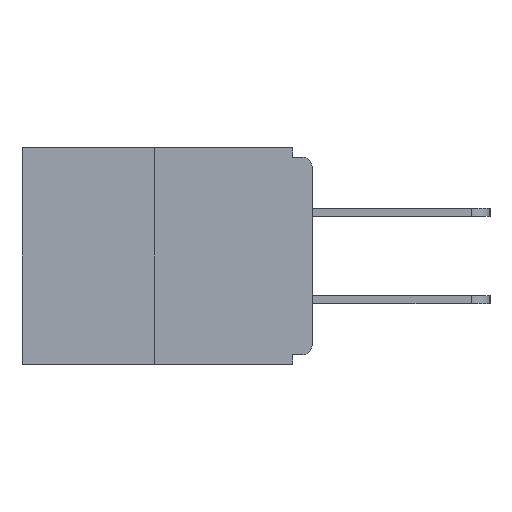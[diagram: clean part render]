
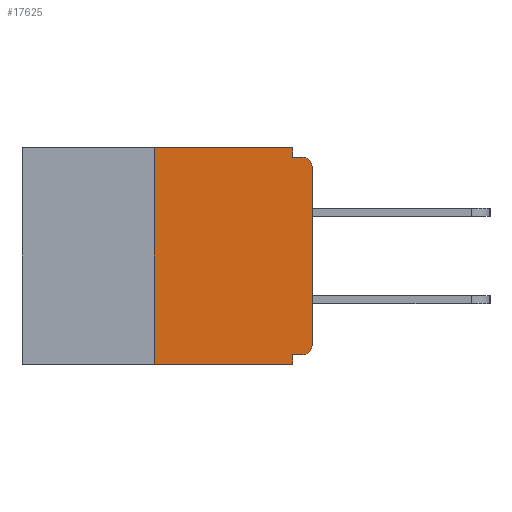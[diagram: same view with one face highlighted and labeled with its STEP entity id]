
A CAD part, left-side view. The second image highlights one B-rep face of the part: STEP entity #17625.
In plain terms, the highlighted planar face has unit normal (-1, 0, 0).
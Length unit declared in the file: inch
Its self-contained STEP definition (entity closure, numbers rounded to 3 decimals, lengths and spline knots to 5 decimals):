
#18 = EDGE_CURVE ( 'NONE', #6038, #10731, #11660, .T. ) ;
#151 = ORIENTED_EDGE ( 'NONE', *, *, #4765, .T. ) ;
#837 = EDGE_CURVE ( 'NONE', #8787, #17537, #17815, .T. ) ;
#917 = CIRCLE ( 'NONE', #1134, 0.015 ) ;
#981 = CARTESIAN_POINT ( 'NONE',  ( 0., 0.031, -0.015 ) ) ;
#1134 = AXIS2_PLACEMENT_3D ( 'NONE', #4329, #6151, #19952 ) ;
#1770 = DIRECTION ( 'NONE',  ( 0., -1., 0. ) ) ;
#2172 = CARTESIAN_POINT ( 'NONE',  ( 0., 0.46, -0.343 ) ) ;
#3503 = ORIENTED_EDGE ( 'NONE', *, *, #23563, .F. ) ;
#3613 = CARTESIAN_POINT ( 'NONE',  ( 0., 0.25, -0.343 ) ) ;
#3852 = CARTESIAN_POINT ( 'NONE',  ( 0., 0.46, 0. ) ) ;
#4032 = DIRECTION ( 'NONE',  ( 0., 0., 1. ) ) ;
#4329 = CARTESIAN_POINT ( 'NONE',  ( 0., 0.015, -0.313 ) ) ;
#4765 = EDGE_CURVE ( 'NONE', #13293, #6038, #917, .T. ) ;
#5050 = CARTESIAN_POINT ( 'NONE',  ( 0., 0.031, 0. ) ) ;
#5633 = DIRECTION ( 'NONE',  ( -1., 0., 0. ) ) ;
#5678 = CARTESIAN_POINT ( 'NONE',  ( 0., 0.015, -0.328 ) ) ;
#5703 = LINE ( 'NONE', #20568, #8484 ) ;
#5723 = EDGE_CURVE ( 'NONE', #21055, #6107, #17226, .T. ) ;
#5806 = EDGE_CURVE ( 'NONE', #13293, #19274, #21233, .T. ) ;
#6010 = CARTESIAN_POINT ( 'NONE',  ( 0., 0.46, 0. ) ) ;
#6038 = VERTEX_POINT ( 'NONE', #20214 ) ;
#6107 = VERTEX_POINT ( 'NONE', #981 ) ;
#6151 = DIRECTION ( 'NONE',  ( -1., 0., 0. ) ) ;
#6972 = DIRECTION ( 'NONE',  ( 0., 0., 1. ) ) ;
#7076 = ORIENTED_EDGE ( 'NONE', *, *, #9445, .F. ) ;
#7399 = CARTESIAN_POINT ( 'NONE',  ( 0., 0.25, 0. ) ) ;
#7522 = CARTESIAN_POINT ( 'NONE',  ( 0., 0., -0.015 ) ) ;
#7923 = VECTOR ( 'NONE', #6972, 39.37008 ) ;
#7946 = DIRECTION ( 'NONE',  ( 0., -1., 0. ) ) ;
#8337 = CARTESIAN_POINT ( 'NONE',  ( 0., 0.031, -0.343 ) ) ;
#8385 = VECTOR ( 'NONE', #7946, 39.37008 ) ;
#8484 = VECTOR ( 'NONE', #16968, 39.37008 ) ;
#8787 = VERTEX_POINT ( 'NONE', #3613 ) ;
#8893 = EDGE_CURVE ( 'NONE', #17537, #21055, #18035, .T. ) ;
#9091 = FACE_OUTER_BOUND ( 'NONE', #11259, .T. ) ;
#9325 = LINE ( 'NONE', #7522, #13367 ) ;
#9394 = DIRECTION ( 'NONE',  ( 0., 1., 0. ) ) ;
#9445 = EDGE_CURVE ( 'NONE', #6107, #10198, #9325, .T. ) ;
#10031 = EDGE_CURVE ( 'NONE', #8787, #23441, #17660, .T. ) ;
#10198 = VERTEX_POINT ( 'NONE', #20001 ) ;
#10731 = VERTEX_POINT ( 'NONE', #18561 ) ;
#10754 = ORIENTED_EDGE ( 'NONE', *, *, #5723, .F. ) ;
#11259 = EDGE_LOOP ( 'NONE', ( #20767, #22901, #16060, #3503, #11901, #151, #18125, #20439, #7076, #10754 ) ) ;
#11642 = CARTESIAN_POINT ( 'NONE',  ( 0., 0.015, -0.03 ) ) ;
#11660 = LINE ( 'NONE', #23448, #17809 ) ;
#11901 = ORIENTED_EDGE ( 'NONE', *, *, #5806, .F. ) ;
#12331 = CARTESIAN_POINT ( 'NONE',  ( 0., 0.031, -0.328 ) ) ;
#12406 = CIRCLE ( 'NONE', #19275, 0.015 ) ;
#12638 = VECTOR ( 'NONE', #9394, 39.37008 ) ;
#13293 = VERTEX_POINT ( 'NONE', #5678 ) ;
#13367 = VECTOR ( 'NONE', #1770, 39.37008 ) ;
#13642 = DIRECTION ( 'NONE',  ( 1., 0., 0. ) ) ;
#15455 = DIRECTION ( 'NONE',  ( 0., 0., -1. ) ) ;
#16060 = ORIENTED_EDGE ( 'NONE', *, *, #10031, .T. ) ;
#16968 = DIRECTION ( 'NONE',  ( 0., 0., -1. ) ) ;
#17226 = LINE ( 'NONE', #5050, #22139 ) ;
#17537 = VERTEX_POINT ( 'NONE', #7399 ) ;
#17625 = ADVANCED_FACE ( 'NONE', ( #9091 ), #23252, .F. ) ;
#17660 = LINE ( 'NONE', #2172, #8385 ) ;
#17809 = VECTOR ( 'NONE', #4032, 39.37008 ) ;
#17815 = LINE ( 'NONE', #19116, #7923 ) ;
#18035 = LINE ( 'NONE', #6010, #18920 ) ;
#18125 = ORIENTED_EDGE ( 'NONE', *, *, #18, .T. ) ;
#18561 = CARTESIAN_POINT ( 'NONE',  ( 0., 0., -0.03 ) ) ;
#18920 = VECTOR ( 'NONE', #25535, 39.37008 ) ;
#19116 = CARTESIAN_POINT ( 'NONE',  ( 0., 0.25, 0. ) ) ;
#19274 = VERTEX_POINT ( 'NONE', #12331 ) ;
#19275 = AXIS2_PLACEMENT_3D ( 'NONE', #11642, #5633, #23577 ) ;
#19952 = DIRECTION ( 'NONE',  ( 0., 0., -1. ) ) ;
#20001 = CARTESIAN_POINT ( 'NONE',  ( 0., 0.015, -0.015 ) ) ;
#20214 = CARTESIAN_POINT ( 'NONE',  ( 0., 0., -0.313 ) ) ;
#20439 = ORIENTED_EDGE ( 'NONE', *, *, #25054, .T. ) ;
#20568 = CARTESIAN_POINT ( 'NONE',  ( 0., 0.031, -0.343 ) ) ;
#20767 = ORIENTED_EDGE ( 'NONE', *, *, #8893, .F. ) ;
#21055 = VERTEX_POINT ( 'NONE', #24094 ) ;
#21233 = LINE ( 'NONE', #23014, #12638 ) ;
#22139 = VECTOR ( 'NONE', #22669, 39.37008 ) ;
#22669 = DIRECTION ( 'NONE',  ( 0., 0., -1. ) ) ;
#22901 = ORIENTED_EDGE ( 'NONE', *, *, #837, .F. ) ;
#23014 = CARTESIAN_POINT ( 'NONE',  ( 0., 0., -0.328 ) ) ;
#23252 = PLANE ( 'NONE',  #23438 ) ;
#23438 = AXIS2_PLACEMENT_3D ( 'NONE', #3852, #13642, #15455 ) ;
#23441 = VERTEX_POINT ( 'NONE', #8337 ) ;
#23448 = CARTESIAN_POINT ( 'NONE',  ( 0., 0., 0. ) ) ;
#23563 = EDGE_CURVE ( 'NONE', #19274, #23441, #5703, .T. ) ;
#23577 = DIRECTION ( 'NONE',  ( 0., 0., -1. ) ) ;
#24094 = CARTESIAN_POINT ( 'NONE',  ( 0., 0.031, 0. ) ) ;
#25054 = EDGE_CURVE ( 'NONE', #10731, #10198, #12406, .T. ) ;
#25535 = DIRECTION ( 'NONE',  ( 0., -1., 0. ) ) ;
